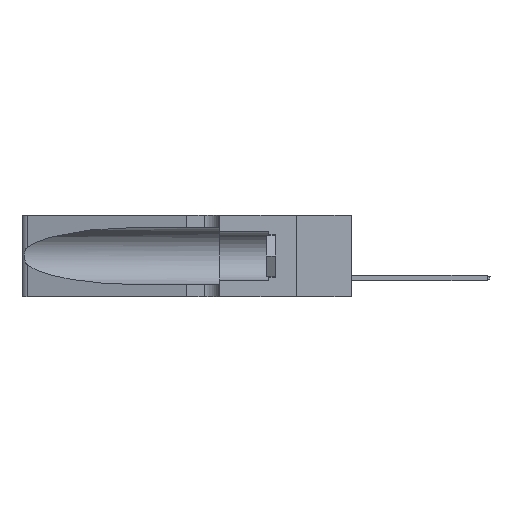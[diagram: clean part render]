
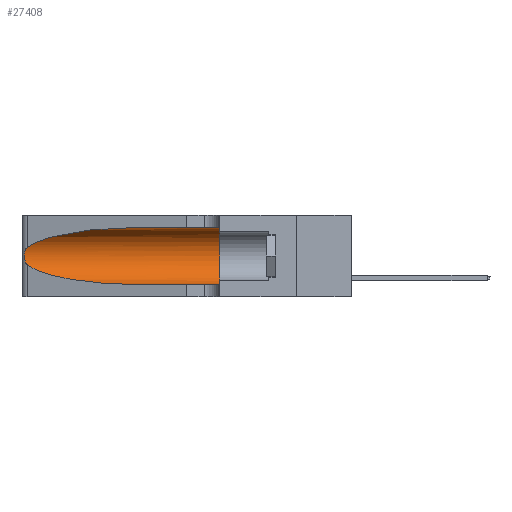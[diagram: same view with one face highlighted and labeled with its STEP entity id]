
A CAD part, left-side view. The second image highlights one B-rep face of the part: STEP entity #27408.
In plain terms, the highlighted cylindrical face has radius 3.308 mm (diameter 6.617 mm), a partial arc.
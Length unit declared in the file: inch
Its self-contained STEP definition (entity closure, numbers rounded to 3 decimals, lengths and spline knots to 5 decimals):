
#428 =( BOUNDED_CURVE ( )  B_SPLINE_CURVE ( 3, ( #27627, #18345, #30077, #21041 ),
 .UNSPECIFIED., .F., .T. ) 
 B_SPLINE_CURVE_WITH_KNOTS ( ( 4, 4 ),
 ( 3.44316, 4.71239 ),
 .UNSPECIFIED. ) 
 CURVE ( )  GEOMETRIC_REPRESENTATION_ITEM ( )  RATIONAL_B_SPLINE_CURVE ( ( 1., 0.87, 0.87, 1. ) ) 
 REPRESENTATION_ITEM ( '' )  );
#444 = CARTESIAN_POINT ( 'NONE',  ( 0.25487, 1.22718, 0.22369 ) ) ;
#1247 = EDGE_CURVE ( 'NONE', #26275, #23308, #4248, .T. ) ;
#2290 = CARTESIAN_POINT ( 'NONE',  ( 0.26018, 1.23835, 0.19895 ) ) ;
#3119 = CARTESIAN_POINT ( 'NONE',  ( 0.25487, 1.22718, 0.14631 ) ) ;
#3200 = CARTESIAN_POINT ( 'NONE',  ( 0.1305, 1.61858, 0.31525 ) ) ;
#3337 = CARTESIAN_POINT ( 'NONE',  ( 0.1305, 0.72297, 0.05475 ) ) ;
#3879 = CARTESIAN_POINT ( 'NONE',  ( 0.2373, 1.15595, 0.28018 ) ) ;
#4050 = CARTESIAN_POINT ( 'NONE',  ( 0.25487, 1.22718, 0.14631 ) ) ;
#4248 = LINE ( 'NONE', #9949, #12651 ) ;
#4324 = CARTESIAN_POINT ( 'NONE',  ( 0.25787, 1.23484, 0.2124 ) ) ;
#6650 = ORIENTED_EDGE ( 'NONE', *, *, #1247, .T. ) ;
#7026 = EDGE_LOOP ( 'NONE', ( #9414, #9611, #29898, #6650, #8587, #8134 ) ) ;
#7909 = DIRECTION ( 'NONE',  ( 0., -1., 0. ) ) ;
#8134 = ORIENTED_EDGE ( 'NONE', *, *, #14011, .F. ) ;
#8587 = ORIENTED_EDGE ( 'NONE', *, *, #14257, .F. ) ;
#9414 = ORIENTED_EDGE ( 'NONE', *, *, #28372, .T. ) ;
#9611 = ORIENTED_EDGE ( 'NONE', *, *, #21142, .T. ) ;
#9949 = CARTESIAN_POINT ( 'NONE',  ( 0.1305, 1.61858, 0.05475 ) ) ;
#10631 = CARTESIAN_POINT ( 'NONE',  ( 0.18966, 0.96281, 0.31525 ) ) ;
#11785 = DIRECTION ( 'NONE',  ( 0., -1., 0. ) ) ;
#12339 = VERTEX_POINT ( 'NONE', #17580 ) ;
#12651 = VECTOR ( 'NONE', #7909, 39.37008 ) ;
#14011 = EDGE_CURVE ( 'NONE', #27359, #23565, #19334, .T. ) ;
#14210 = CARTESIAN_POINT ( 'NONE',  ( 0.26075, 1.23896, 0.178 ) ) ;
#14257 = EDGE_CURVE ( 'NONE', #23565, #23308, #22261, .T. ) ;
#15934 = CARTESIAN_POINT ( 'NONE',  ( 0.25555, 1.22994, 0.2215 ) ) ;
#17256 = CARTESIAN_POINT ( 'NONE',  ( 0.25789, 1.23486, 0.15765 ) ) ;
#17579 = DIRECTION ( 'NONE',  ( 0., 0., 1. ) ) ;
#17580 = CARTESIAN_POINT ( 'NONE',  ( 0.25487, 1.22718, 0.22369 ) ) ;
#18052 = VERTEX_POINT ( 'NONE', #4050 ) ;
#18345 = CARTESIAN_POINT ( 'NONE',  ( 0.2373, 1.15595, 0.08982 ) ) ;
#18707 = CARTESIAN_POINT ( 'NONE',  ( 0.25856, 1.23593, 0.16098 ) ) ;
#19334 = LINE ( 'NONE', #3200, #23326 ) ;
#19433 = B_SPLINE_CURVE_WITH_KNOTS ( 'NONE', 3,
 ( #444, #15934, #22924, #4324, #27226, #2290, #25676, #14210, #20779, #18707, #17256, #21533, #28644, #3119 ),
 .UNSPECIFIED., .F., .F.,
 ( 4, 2, 2, 2, 2, 2, 4 ),
 ( 0., 0.00027, 0.00053, 0.00107, 0.0016, 0.00187, 0.00214 ),
 .UNSPECIFIED. ) ;
#19617 = CARTESIAN_POINT ( 'NONE',  ( 0.1305, 1.61858, 0.185 ) ) ;
#20779 = CARTESIAN_POINT ( 'NONE',  ( 0.26017, 1.23833, 0.17102 ) ) ;
#21041 = CARTESIAN_POINT ( 'NONE',  ( 0.1305, 0.72297, 0.05475 ) ) ;
#21142 = EDGE_CURVE ( 'NONE', #12339, #18052, #19433, .T. ) ;
#21533 = CARTESIAN_POINT ( 'NONE',  ( 0.25639, 1.23186, 0.15144 ) ) ;
#21977 = DIRECTION ( 'NONE',  ( 0., 0., -1. ) ) ;
#22261 = CIRCLE ( 'NONE', #26154, 0.13025 ) ;
#22542 = CYLINDRICAL_SURFACE ( 'NONE', #25207, 0.13025 ) ;
#22924 = CARTESIAN_POINT ( 'NONE',  ( 0.25639, 1.23184, 0.21858 ) ) ;
#23308 = VERTEX_POINT ( 'NONE', #25287 ) ;
#23316 = EDGE_CURVE ( 'NONE', #18052, #26275, #428, .T. ) ;
#23326 = VECTOR ( 'NONE', #11785, 39.37008 ) ;
#23517 =( BOUNDED_CURVE ( )  B_SPLINE_CURVE ( 3, ( #24527, #10631, #3879, #24731 ),
 .UNSPECIFIED., .F., .T. ) 
 B_SPLINE_CURVE_WITH_KNOTS ( ( 4, 4 ),
 ( 1.5708, 2.84003 ),
 .UNSPECIFIED. ) 
 CURVE ( )  GEOMETRIC_REPRESENTATION_ITEM ( )  RATIONAL_B_SPLINE_CURVE ( ( 1., 0.87, 0.87, 1. ) ) 
 REPRESENTATION_ITEM ( '' )  );
#23565 = VERTEX_POINT ( 'NONE', #25997 ) ;
#24311 = DIRECTION ( 'NONE',  ( 0., -1., 0. ) ) ;
#24497 = CARTESIAN_POINT ( 'NONE',  ( 0.1305, 0.35, 0.185 ) ) ;
#24527 = CARTESIAN_POINT ( 'NONE',  ( 0.1305, 0.72297, 0.31525 ) ) ;
#24731 = CARTESIAN_POINT ( 'NONE',  ( 0.25487, 1.22718, 0.22369 ) ) ;
#25207 = AXIS2_PLACEMENT_3D ( 'NONE', #19617, #24311, #21977 ) ;
#25287 = CARTESIAN_POINT ( 'NONE',  ( 0.1305, 0.35, 0.05475 ) ) ;
#25482 = FACE_OUTER_BOUND ( 'NONE', #7026, .T. ) ;
#25676 = CARTESIAN_POINT ( 'NONE',  ( 0.26075, 1.23896, 0.19203 ) ) ;
#25997 = CARTESIAN_POINT ( 'NONE',  ( 0.1305, 0.35, 0.31525 ) ) ;
#26154 = AXIS2_PLACEMENT_3D ( 'NONE', #24497, #29358, #17579 ) ;
#26275 = VERTEX_POINT ( 'NONE', #3337 ) ;
#26675 = CARTESIAN_POINT ( 'NONE',  ( 0.1305, 0.72297, 0.31525 ) ) ;
#27226 = CARTESIAN_POINT ( 'NONE',  ( 0.25854, 1.2359, 0.20912 ) ) ;
#27359 = VERTEX_POINT ( 'NONE', #26675 ) ;
#27408 = ADVANCED_FACE ( 'NONE', ( #25482 ), #22542, .F. ) ;
#27627 = CARTESIAN_POINT ( 'NONE',  ( 0.25487, 1.22718, 0.14631 ) ) ;
#28372 = EDGE_CURVE ( 'NONE', #27359, #12339, #23517, .T. ) ;
#28644 = CARTESIAN_POINT ( 'NONE',  ( 0.25555, 1.22993, 0.14849 ) ) ;
#29358 = DIRECTION ( 'NONE',  ( 0., 1., 0. ) ) ;
#29898 = ORIENTED_EDGE ( 'NONE', *, *, #23316, .T. ) ;
#30077 = CARTESIAN_POINT ( 'NONE',  ( 0.18966, 0.96281, 0.05475 ) ) ;
